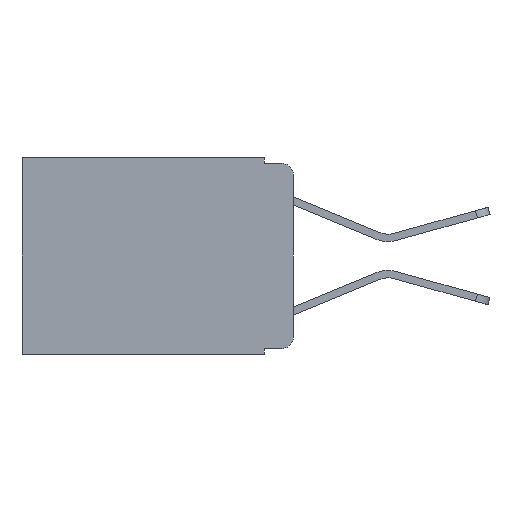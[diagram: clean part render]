
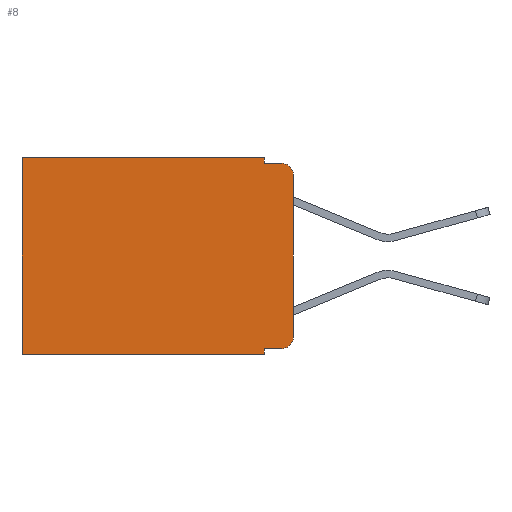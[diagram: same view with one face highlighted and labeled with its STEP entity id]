
A CAD part, left-side view. The second image highlights one B-rep face of the part: STEP entity #8.
In plain terms, the highlighted planar face has unit normal (-1, 0, 0).
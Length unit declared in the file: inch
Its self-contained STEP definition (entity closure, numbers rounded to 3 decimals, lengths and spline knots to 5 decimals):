
#8 = ADVANCED_FACE ( 'NONE', ( #8698 ), #7211, .F. ) ;
#410 = ORIENTED_EDGE ( 'NONE', *, *, #3227, .F. ) ;
#923 = ORIENTED_EDGE ( 'NONE', *, *, #5521, .F. ) ;
#1183 = CARTESIAN_POINT ( 'NONE',  ( 0.298, 0.02, -0.313 ) ) ;
#1285 = CIRCLE ( 'NONE', #16157, 0.02 ) ;
#1358 = LINE ( 'NONE', #11732, #9252 ) ;
#1399 = EDGE_CURVE ( 'NONE', #5498, #2829, #1449, .T. ) ;
#1408 = EDGE_CURVE ( 'NONE', #7582, #10625, #1358, .T. ) ;
#1420 = LINE ( 'NONE', #16871, #10636 ) ;
#1449 = LINE ( 'NONE', #11644, #11451 ) ;
#1683 = DIRECTION ( 'NONE',  ( 0., 0., -1. ) ) ;
#1933 = ORIENTED_EDGE ( 'NONE', *, *, #10104, .F. ) ;
#2309 = ORIENTED_EDGE ( 'NONE', *, *, #17834, .T. ) ;
#2829 = VERTEX_POINT ( 'NONE', #16803 ) ;
#2872 = CIRCLE ( 'NONE', #13612, 0.02 ) ;
#2940 = DIRECTION ( 'NONE',  ( 0., 0., -1. ) ) ;
#3097 = CARTESIAN_POINT ( 'NONE',  ( 0.298, 0.473, 0. ) ) ;
#3227 = EDGE_CURVE ( 'NONE', #2829, #16460, #19348, .T. ) ;
#3466 = ORIENTED_EDGE ( 'NONE', *, *, #1399, .F. ) ;
#3587 = VECTOR ( 'NONE', #9541, 39.37008 ) ;
#3907 = LINE ( 'NONE', #5505, #4371 ) ;
#4344 = DIRECTION ( 'NONE',  ( 0., 0., -1. ) ) ;
#4371 = VECTOR ( 'NONE', #15906, 39.37008 ) ;
#4472 = DIRECTION ( 'NONE',  ( -1., 0., 0. ) ) ;
#4592 = VECTOR ( 'NONE', #4344, 39.37008 ) ;
#5313 = CARTESIAN_POINT ( 'NONE',  ( 0.298, 0.02, -0.333 ) ) ;
#5416 = VECTOR ( 'NONE', #17727, 39.37008 ) ;
#5498 = VERTEX_POINT ( 'NONE', #8645 ) ;
#5505 = CARTESIAN_POINT ( 'NONE',  ( 0.298, 0., 0. ) ) ;
#5521 = EDGE_CURVE ( 'NONE', #14667, #5526, #3907, .T. ) ;
#5526 = VERTEX_POINT ( 'NONE', #11320 ) ;
#5750 = DIRECTION ( 'NONE',  ( 0., 0., -1. ) ) ;
#5922 = DIRECTION ( 'NONE',  ( 0., -1., 0. ) ) ;
#5927 = CARTESIAN_POINT ( 'NONE',  ( 0.298, 0., 0. ) ) ;
#6107 = CARTESIAN_POINT ( 'NONE',  ( 0.298, 0.02, -0.01 ) ) ;
#7211 = PLANE ( 'NONE',  #14827 ) ;
#7222 = DIRECTION ( 'NONE',  ( -1., 0., 0. ) ) ;
#7315 = EDGE_CURVE ( 'NONE', #13129, #8223, #14386, .T. ) ;
#7368 = DIRECTION ( 'NONE',  ( 0., 1., 0. ) ) ;
#7441 = CARTESIAN_POINT ( 'NONE',  ( 0.298, 0.02, -0.03 ) ) ;
#7582 = VERTEX_POINT ( 'NONE', #17937 ) ;
#7789 = LINE ( 'NONE', #12322, #4592 ) ;
#8223 = VERTEX_POINT ( 'NONE', #9879 ) ;
#8519 = CARTESIAN_POINT ( 'NONE',  ( 0.298, 0.473, 0. ) ) ;
#8645 = CARTESIAN_POINT ( 'NONE',  ( 0.298, 0.051, 0. ) ) ;
#8698 = FACE_OUTER_BOUND ( 'NONE', #18441, .T. ) ;
#9252 = VECTOR ( 'NONE', #5922, 39.37008 ) ;
#9279 = ORIENTED_EDGE ( 'NONE', *, *, #18168, .T. ) ;
#9541 = DIRECTION ( 'NONE',  ( 0., -1., 0. ) ) ;
#9879 = CARTESIAN_POINT ( 'NONE',  ( 0.298, 0.473, -0.343 ) ) ;
#10104 = EDGE_CURVE ( 'NONE', #7582, #13129, #7789, .T. ) ;
#10113 = LINE ( 'NONE', #8519, #5416 ) ;
#10256 = CARTESIAN_POINT ( 'NONE',  ( 0.298, 0.051, -0.01 ) ) ;
#10625 = VERTEX_POINT ( 'NONE', #5313 ) ;
#10636 = VECTOR ( 'NONE', #7368, 39.37008 ) ;
#11206 = CARTESIAN_POINT ( 'NONE',  ( 0.298, 0., -0.343 ) ) ;
#11320 = CARTESIAN_POINT ( 'NONE',  ( 0.298, 0., -0.313 ) ) ;
#11451 = VECTOR ( 'NONE', #16411, 39.37008 ) ;
#11644 = CARTESIAN_POINT ( 'NONE',  ( 0.298, 0.051, 0. ) ) ;
#11732 = CARTESIAN_POINT ( 'NONE',  ( 0.298, 0.051, -0.333 ) ) ;
#12032 = CARTESIAN_POINT ( 'NONE',  ( 0.298, 0., -0.03 ) ) ;
#12322 = CARTESIAN_POINT ( 'NONE',  ( 0.298, 0.051, 0. ) ) ;
#12642 = ORIENTED_EDGE ( 'NONE', *, *, #13385, .T. ) ;
#13023 = VECTOR ( 'NONE', #18845, 39.37008 ) ;
#13101 = CARTESIAN_POINT ( 'NONE',  ( 0.298, 0.051, -0.343 ) ) ;
#13129 = VERTEX_POINT ( 'NONE', #13101 ) ;
#13261 = VERTEX_POINT ( 'NONE', #3097 ) ;
#13385 = EDGE_CURVE ( 'NONE', #5498, #13261, #1420, .T. ) ;
#13487 = ORIENTED_EDGE ( 'NONE', *, *, #17586, .T. ) ;
#13612 = AXIS2_PLACEMENT_3D ( 'NONE', #1183, #7222, #5750 ) ;
#14386 = LINE ( 'NONE', #11206, #13023 ) ;
#14667 = VERTEX_POINT ( 'NONE', #12032 ) ;
#14827 = AXIS2_PLACEMENT_3D ( 'NONE', #5927, #17908, #2940 ) ;
#15833 = ORIENTED_EDGE ( 'NONE', *, *, #7315, .F. ) ;
#15906 = DIRECTION ( 'NONE',  ( 0., 0., -1. ) ) ;
#16157 = AXIS2_PLACEMENT_3D ( 'NONE', #7441, #4472, #1683 ) ;
#16411 = DIRECTION ( 'NONE',  ( 0., 0., -1. ) ) ;
#16460 = VERTEX_POINT ( 'NONE', #6107 ) ;
#16803 = CARTESIAN_POINT ( 'NONE',  ( 0.298, 0.051, -0.01 ) ) ;
#16871 = CARTESIAN_POINT ( 'NONE',  ( 0.298, 0., 0. ) ) ;
#17190 = ORIENTED_EDGE ( 'NONE', *, *, #1408, .T. ) ;
#17586 = EDGE_CURVE ( 'NONE', #13261, #8223, #10113, .T. ) ;
#17727 = DIRECTION ( 'NONE',  ( 0., 0., -1. ) ) ;
#17834 = EDGE_CURVE ( 'NONE', #14667, #16460, #1285, .T. ) ;
#17908 = DIRECTION ( 'NONE',  ( 1., 0., 0. ) ) ;
#17937 = CARTESIAN_POINT ( 'NONE',  ( 0.298, 0.051, -0.333 ) ) ;
#18168 = EDGE_CURVE ( 'NONE', #10625, #5526, #2872, .T. ) ;
#18441 = EDGE_LOOP ( 'NONE', ( #923, #2309, #410, #3466, #12642, #13487, #15833, #1933, #17190, #9279 ) ) ;
#18845 = DIRECTION ( 'NONE',  ( 0., 1., 0. ) ) ;
#19348 = LINE ( 'NONE', #10256, #3587 ) ;
